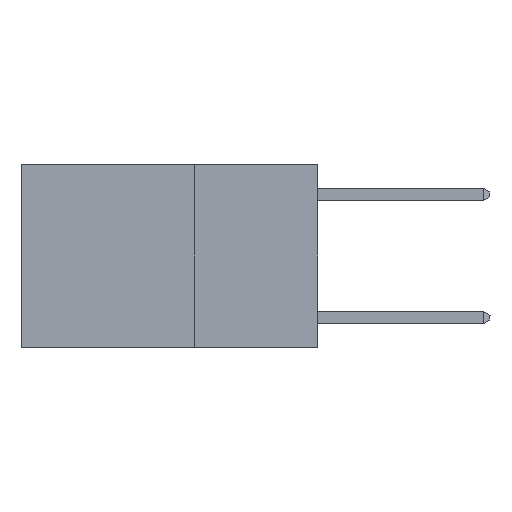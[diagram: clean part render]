
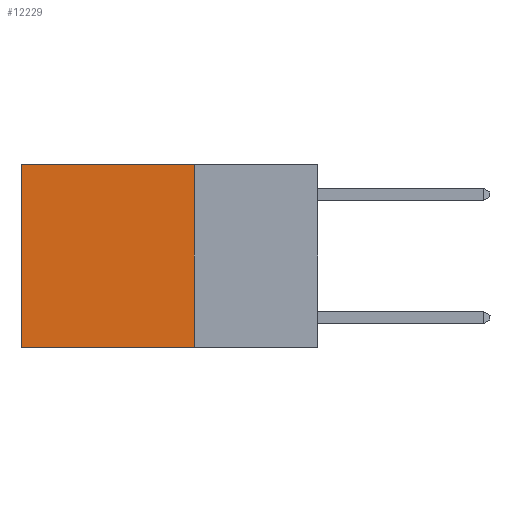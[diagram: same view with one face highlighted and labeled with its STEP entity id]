
A CAD part, left-side view. The second image highlights one B-rep face of the part: STEP entity #12229.
In plain terms, the highlighted planar face has unit normal (-1, 0, 0).
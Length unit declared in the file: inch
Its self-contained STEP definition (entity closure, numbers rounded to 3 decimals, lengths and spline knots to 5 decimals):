
#164 = DIRECTION ( 'NONE',  ( 0., 1., 0. ) ) ;
#480 = LINE ( 'NONE', #1612, #3051 ) ;
#903 = CARTESIAN_POINT ( 'NONE',  ( 0.2625, 0.25, -0.37 ) ) ;
#1291 = VERTEX_POINT ( 'NONE', #7779 ) ;
#1494 = PLANE ( 'NONE',  #7706 ) ;
#1612 = CARTESIAN_POINT ( 'NONE',  ( 0.2625, 0.6, 0. ) ) ;
#1682 = VERTEX_POINT ( 'NONE', #5834 ) ;
#2038 = VERTEX_POINT ( 'NONE', #8711 ) ;
#2508 = CARTESIAN_POINT ( 'NONE',  ( 0.2625, 0.25, 0. ) ) ;
#3051 = VECTOR ( 'NONE', #4603, 39.37008 ) ;
#3174 = ORIENTED_EDGE ( 'NONE', *, *, #7635, .F. ) ;
#4039 = EDGE_CURVE ( 'NONE', #1682, #9270, #480, .T. ) ;
#4250 = EDGE_CURVE ( 'NONE', #1291, #1682, #10653, .T. ) ;
#4603 = DIRECTION ( 'NONE',  ( 0., 0., -1. ) ) ;
#5736 = FACE_OUTER_BOUND ( 'NONE', #5858, .T. ) ;
#5834 = CARTESIAN_POINT ( 'NONE',  ( 0.2625, 0.6, 0. ) ) ;
#5858 = EDGE_LOOP ( 'NONE', ( #6662, #12153, #3174, #9851 ) ) ;
#6473 = LINE ( 'NONE', #903, #8781 ) ;
#6615 = LINE ( 'NONE', #12413, #7685 ) ;
#6662 = ORIENTED_EDGE ( 'NONE', *, *, #4039, .T. ) ;
#7056 = EDGE_CURVE ( 'NONE', #2038, #9270, #6473, .T. ) ;
#7635 = EDGE_CURVE ( 'NONE', #1291, #2038, #6615, .T. ) ;
#7685 = VECTOR ( 'NONE', #7762, 39.37008 ) ;
#7690 = DIRECTION ( 'NONE',  ( 0., 1., 0. ) ) ;
#7706 = AXIS2_PLACEMENT_3D ( 'NONE', #2508, #11284, #12265 ) ;
#7762 = DIRECTION ( 'NONE',  ( 0., 0., -1. ) ) ;
#7774 = CARTESIAN_POINT ( 'NONE',  ( 0.2625, 0.25, 0. ) ) ;
#7779 = CARTESIAN_POINT ( 'NONE',  ( 0.2625, 0.25, 0. ) ) ;
#8080 = VECTOR ( 'NONE', #164, 39.37008 ) ;
#8711 = CARTESIAN_POINT ( 'NONE',  ( 0.2625, 0.25, -0.37 ) ) ;
#8781 = VECTOR ( 'NONE', #7690, 39.37008 ) ;
#9270 = VERTEX_POINT ( 'NONE', #9554 ) ;
#9554 = CARTESIAN_POINT ( 'NONE',  ( 0.2625, 0.6, -0.37 ) ) ;
#9851 = ORIENTED_EDGE ( 'NONE', *, *, #4250, .T. ) ;
#10653 = LINE ( 'NONE', #7774, #8080 ) ;
#11284 = DIRECTION ( 'NONE',  ( 1., 0., 0. ) ) ;
#12153 = ORIENTED_EDGE ( 'NONE', *, *, #7056, .F. ) ;
#12229 = ADVANCED_FACE ( 'NONE', ( #5736 ), #1494, .F. ) ;
#12265 = DIRECTION ( 'NONE',  ( 0., 0., -1. ) ) ;
#12413 = CARTESIAN_POINT ( 'NONE',  ( 0.2625, 0.25, 0. ) ) ;
